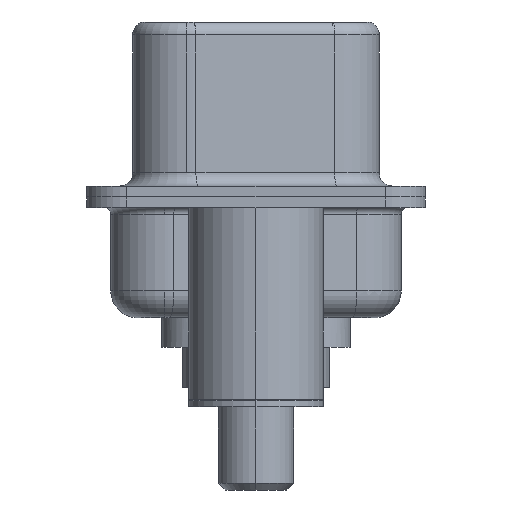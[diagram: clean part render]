
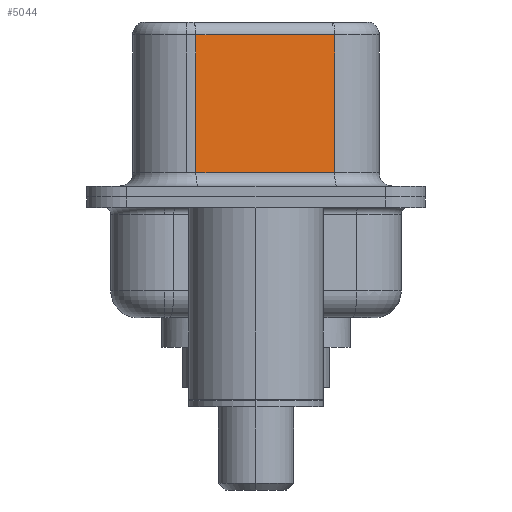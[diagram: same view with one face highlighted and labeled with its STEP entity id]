
A CAD part, left-side view. The second image highlights one B-rep face of the part: STEP entity #5044.
In plain terms, the highlighted planar face has unit normal (-0.985, -0.174, 0).
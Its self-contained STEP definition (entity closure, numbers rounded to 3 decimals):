
#235 = VECTOR ( 'NONE', #10350, 1000. ) ;
#1004 = CARTESIAN_POINT ( 'NONE',  ( 3.67, 2.233, 0.9 ) ) ;
#1834 = CARTESIAN_POINT ( 'NONE',  ( 4.58, -2.927, 6.02 ) ) ;
#1849 = CARTESIAN_POINT ( 'NONE',  ( 4.58, -2.927, 0.9 ) ) ;
#2223 = EDGE_CURVE ( 'NONE', #8956, #11947, #16814, .T. ) ;
#3133 = CARTESIAN_POINT ( 'NONE',  ( 4.58, -2.927, 6.52 ) ) ;
#3738 = AXIS2_PLACEMENT_3D ( 'NONE', #14330, #19116, #14477 ) ;
#4396 = LINE ( 'NONE', #12143, #235 ) ;
#4730 = CARTESIAN_POINT ( 'NONE',  ( 3.67, 2.233, 6.52 ) ) ;
#5044 = ADVANCED_FACE ( 'NONE', ( #14192 ), #19176, .F. ) ;
#6170 = LINE ( 'NONE', #3133, #18488 ) ;
#6670 = EDGE_CURVE ( 'NONE', #11947, #20023, #4396, .T. ) ;
#6882 = LINE ( 'NONE', #12999, #7121 ) ;
#7121 = VECTOR ( 'NONE', #19388, 1000. ) ;
#7762 = EDGE_CURVE ( 'NONE', #15133, #20023, #6170, .T. ) ;
#8956 = VERTEX_POINT ( 'NONE', #18072 ) ;
#9094 = EDGE_CURVE ( 'NONE', #15133, #8956, #6882, .T. ) ;
#9477 = DIRECTION ( 'NONE',  ( 0., 0., -1. ) ) ;
#9568 = ORIENTED_EDGE ( 'NONE', *, *, #7762, .F. ) ;
#10350 = DIRECTION ( 'NONE',  ( 0.174, -0.985, 0. ) ) ;
#10435 = ORIENTED_EDGE ( 'NONE', *, *, #2223, .T. ) ;
#11096 = VECTOR ( 'NONE', #19454, 1000. ) ;
#11947 = VERTEX_POINT ( 'NONE', #1004 ) ;
#11998 = EDGE_LOOP ( 'NONE', ( #9568, #18575, #10435, #17260 ) ) ;
#12143 = CARTESIAN_POINT ( 'NONE',  ( 4.58, -2.927, 0.9 ) ) ;
#12999 = CARTESIAN_POINT ( 'NONE',  ( 4.58, -2.927, 6.02 ) ) ;
#14192 = FACE_OUTER_BOUND ( 'NONE', #11998, .T. ) ;
#14330 = CARTESIAN_POINT ( 'NONE',  ( 4.58, -2.927, 6.52 ) ) ;
#14477 = DIRECTION ( 'NONE',  ( -0.174, 0.985, 0. ) ) ;
#15133 = VERTEX_POINT ( 'NONE', #1834 ) ;
#16814 = LINE ( 'NONE', #4730, #11096 ) ;
#17260 = ORIENTED_EDGE ( 'NONE', *, *, #6670, .T. ) ;
#18072 = CARTESIAN_POINT ( 'NONE',  ( 3.67, 2.233, 6.02 ) ) ;
#18488 = VECTOR ( 'NONE', #9477, 1000. ) ;
#18575 = ORIENTED_EDGE ( 'NONE', *, *, #9094, .T. ) ;
#19116 = DIRECTION ( 'NONE',  ( 0.985, 0.174, 0. ) ) ;
#19176 = PLANE ( 'NONE',  #3738 ) ;
#19388 = DIRECTION ( 'NONE',  ( -0.174, 0.985, 0. ) ) ;
#19454 = DIRECTION ( 'NONE',  ( 0., 0., -1. ) ) ;
#20023 = VERTEX_POINT ( 'NONE', #1849 ) ;
